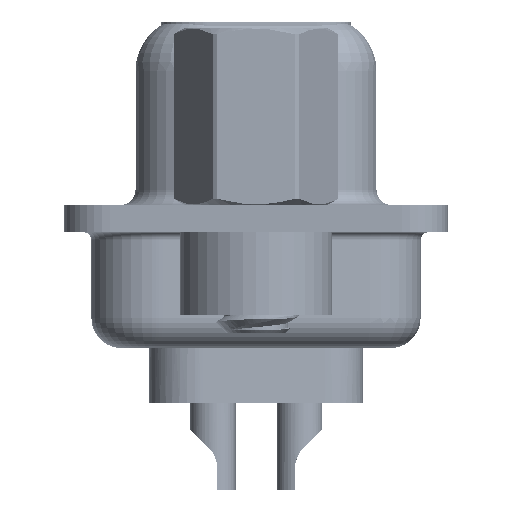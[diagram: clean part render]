
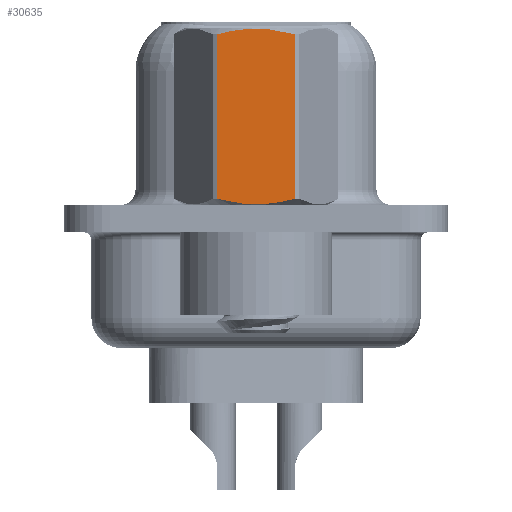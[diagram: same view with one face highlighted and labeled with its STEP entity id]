
A CAD part, left-side view. The second image highlights one B-rep face of the part: STEP entity #30635.
In plain terms, the highlighted planar face has unit normal (-1, 0, 0).
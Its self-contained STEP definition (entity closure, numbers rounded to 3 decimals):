
#591 = DIRECTION ( 'NONE',  ( 0., 0., -1. ) ) ;
#1278 = EDGE_CURVE ( 'NONE', #3290, #4426, #5129, .T. ) ;
#1322 = CARTESIAN_POINT ( 'NONE',  ( -2.381, -1.066, 0.596 ) ) ;
#1588 = CARTESIAN_POINT ( 'NONE',  ( -2.381, 0.215, 6.232 ) ) ;
#3094 = DIRECTION ( 'NONE',  ( 0., 0., 1. ) ) ;
#3290 = VERTEX_POINT ( 'NONE', #16640 ) ;
#3309 = CARTESIAN_POINT ( 'NONE',  ( -2.381, 1.273, 3.792 ) ) ;
#4165 = CARTESIAN_POINT ( 'NONE',  ( -2.381, -1.066, 6.104 ) ) ;
#4270 = CARTESIAN_POINT ( 'NONE',  ( -2.381, 0.853, 6.151 ) ) ;
#4426 = VERTEX_POINT ( 'NONE', #26150 ) ;
#4466 = VECTOR ( 'NONE', #591, 1000. ) ;
#5129 = LINE ( 'NONE', #8601, #12979 ) ;
#5572 = B_SPLINE_CURVE_WITH_KNOTS ( 'NONE', 3,
 ( #9523, #4165, #14769, #33179, #17358, #1588, #20013, #4270, #22640, #7008 ),
 .UNSPECIFIED., .F., .F.,
 ( 4, 2, 2, 2, 4 ),
 ( 0.001, 0.002, 0.002, 0.003, 0.004 ),
 .UNSPECIFIED. ) ;
#6729 = PLANE ( 'NONE',  #34239 ) ;
#7008 = CARTESIAN_POINT ( 'NONE',  ( -2.381, 1.273, 6.048 ) ) ;
#7335 = ORIENTED_EDGE ( 'NONE', *, *, #18209, .T. ) ;
#8601 = CARTESIAN_POINT ( 'NONE',  ( -2.381, -1.273, 3.792 ) ) ;
#8997 = ORIENTED_EDGE ( 'NONE', *, *, #24145, .T. ) ;
#9285 = CARTESIAN_POINT ( 'NONE',  ( -2.381, 1.273, 0.652 ) ) ;
#9368 = CARTESIAN_POINT ( 'NONE',  ( -2.381, 1.375, -3.75 ) ) ;
#9523 = CARTESIAN_POINT ( 'NONE',  ( -2.381, -1.273, 6.048 ) ) ;
#11930 = CARTESIAN_POINT ( 'NONE',  ( -2.381, 0.428, 0.485 ) ) ;
#12020 = DIRECTION ( 'NONE',  ( 0., -1., 0. ) ) ;
#12349 = LINE ( 'NONE', #3309, #4466 ) ;
#12979 = VECTOR ( 'NONE', #3094, 1000. ) ;
#13588 = ORIENTED_EDGE ( 'NONE', *, *, #21414, .T. ) ;
#14526 = CARTESIAN_POINT ( 'NONE',  ( -2.381, -0.215, 0.468 ) ) ;
#14769 = CARTESIAN_POINT ( 'NONE',  ( -2.381, -0.858, 6.15 ) ) ;
#14922 = EDGE_LOOP ( 'NONE', ( #7335, #16236, #13588, #8997 ) ) ;
#16236 = ORIENTED_EDGE ( 'NONE', *, *, #1278, .T. ) ;
#16640 = CARTESIAN_POINT ( 'NONE',  ( -2.381, -1.273, 0.652 ) ) ;
#17120 = CARTESIAN_POINT ( 'NONE',  ( -2.381, -0.858, 0.55 ) ) ;
#17358 = CARTESIAN_POINT ( 'NONE',  ( -2.381, -0.215, 6.232 ) ) ;
#18209 = EDGE_CURVE ( 'NONE', #27372, #3290, #26793, .T. ) ;
#19786 = CARTESIAN_POINT ( 'NONE',  ( -2.381, -1.273, 0.652 ) ) ;
#20013 = CARTESIAN_POINT ( 'NONE',  ( -2.381, 0.428, 6.215 ) ) ;
#21414 = EDGE_CURVE ( 'NONE', #4426, #31644, #5572, .T. ) ;
#22640 = CARTESIAN_POINT ( 'NONE',  ( -2.381, 1.065, 6.104 ) ) ;
#24145 = EDGE_CURVE ( 'NONE', #31644, #27372, #12349, .T. ) ;
#24927 = CARTESIAN_POINT ( 'NONE',  ( -2.381, 1.065, 0.596 ) ) ;
#25527 = FACE_OUTER_BOUND ( 'NONE', #14922, .T. ) ;
#26150 = CARTESIAN_POINT ( 'NONE',  ( -2.381, -1.273, 6.048 ) ) ;
#26793 = B_SPLINE_CURVE_WITH_KNOTS ( 'NONE', 3,
 ( #9285, #24927, #27590, #11930, #30194, #14526, #32931, #17120, #1322, #19786 ),
 .UNSPECIFIED., .F., .F.,
 ( 4, 2, 2, 2, 4 ),
 ( 0.003, 0.003, 0.004, 0.004, 0.005 ),
 .UNSPECIFIED. ) ;
#27372 = VERTEX_POINT ( 'NONE', #32904 ) ;
#27590 = CARTESIAN_POINT ( 'NONE',  ( -2.381, 0.853, 0.549 ) ) ;
#27676 = DIRECTION ( 'NONE',  ( -1., 0., 0. ) ) ;
#30194 = CARTESIAN_POINT ( 'NONE',  ( -2.381, 0.215, 0.468 ) ) ;
#30635 = ADVANCED_FACE ( 'NONE', ( #25527 ), #6729, .T. ) ;
#31644 = VERTEX_POINT ( 'NONE', #31867 ) ;
#31867 = CARTESIAN_POINT ( 'NONE',  ( -2.381, 1.273, 6.048 ) ) ;
#32904 = CARTESIAN_POINT ( 'NONE',  ( -2.381, 1.273, 0.652 ) ) ;
#32931 = CARTESIAN_POINT ( 'NONE',  ( -2.381, -0.432, 0.485 ) ) ;
#33179 = CARTESIAN_POINT ( 'NONE',  ( -2.381, -0.432, 6.215 ) ) ;
#34239 = AXIS2_PLACEMENT_3D ( 'NONE', #9368, #27676, #12020 ) ;
